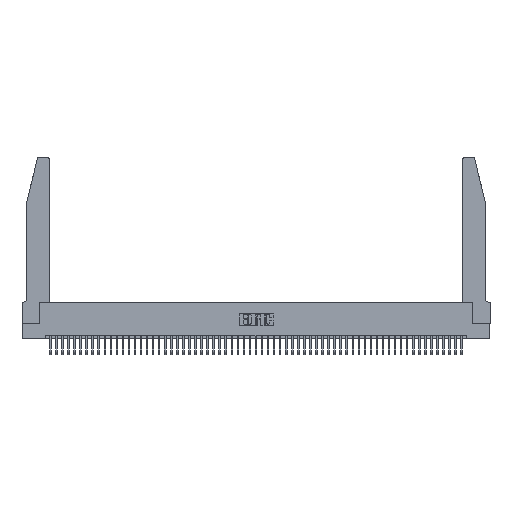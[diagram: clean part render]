
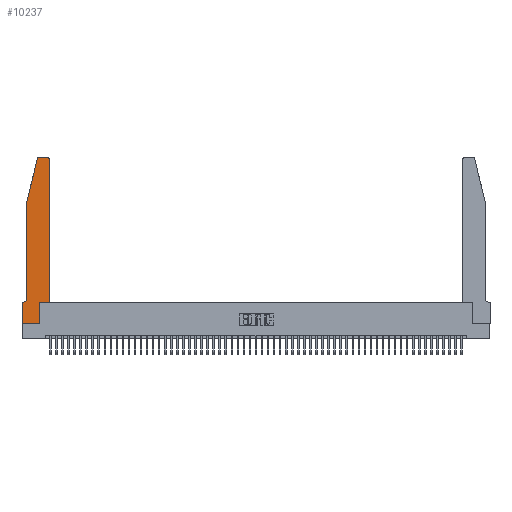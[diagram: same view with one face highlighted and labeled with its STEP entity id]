
A CAD part, top view. The second image highlights one B-rep face of the part: STEP entity #10237.
In plain terms, the highlighted planar face has unit normal (0, 0, 1).
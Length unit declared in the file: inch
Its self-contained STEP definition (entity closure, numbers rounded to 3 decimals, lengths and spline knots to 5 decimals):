
#79 = AXIS2_PLACEMENT_3D ( 'NONE', #24327, #52691, #28423 ) ;
#608 = DIRECTION ( 'NONE',  ( 1., 0., 0. ) ) ;
#946 = DIRECTION ( 'NONE',  ( -1., 0., 0. ) ) ;
#1946 = VERTEX_POINT ( 'NONE', #51150 ) ;
#1989 = EDGE_CURVE ( 'NONE', #50566, #15829, #42300, .T. ) ;
#2062 = VERTEX_POINT ( 'NONE', #47777 ) ;
#3267 = CIRCLE ( 'NONE', #79, 0.03 ) ;
#3657 = VERTEX_POINT ( 'NONE', #42501 ) ;
#4906 = LINE ( 'NONE', #50352, #36424 ) ;
#5288 = VERTEX_POINT ( 'NONE', #52669 ) ;
#5854 = VECTOR ( 'NONE', #33535, 39.37008 ) ;
#5863 = LINE ( 'NONE', #35959, #27805 ) ;
#6526 = VECTOR ( 'NONE', #21671, 39.37008 ) ;
#8458 = ORIENTED_EDGE ( 'NONE', *, *, #50319, .T. ) ;
#8859 = CARTESIAN_POINT ( 'NONE',  ( 0.4205, 2.72, 0.37 ) ) ;
#9174 = CIRCLE ( 'NONE', #15406, 0.07 ) ;
#9323 = EDGE_CURVE ( 'NONE', #41227, #2062, #26548, .T. ) ;
#10237 = ADVANCED_FACE ( 'NONE', ( #10332 ), #19531, .T. ) ;
#10332 = FACE_OUTER_BOUND ( 'NONE', #48337, .T. ) ;
#10875 = VERTEX_POINT ( 'NONE', #20362 ) ;
#11141 = ORIENTED_EDGE ( 'NONE', *, *, #15464, .T. ) ;
#11398 = DIRECTION ( 'NONE',  ( 0., 1., 0. ) ) ;
#11643 = AXIS2_PLACEMENT_3D ( 'NONE', #39808, #47992, #23656 ) ;
#11750 = VECTOR ( 'NONE', #25500, 39.37008 ) ;
#12525 = DIRECTION ( 'NONE',  ( -1., 0., 0. ) ) ;
#13032 = DIRECTION ( 'NONE',  ( 1., 0., 0. ) ) ;
#13220 = CARTESIAN_POINT ( 'NONE',  ( 0., 0., 0.37 ) ) ;
#13730 = ORIENTED_EDGE ( 'NONE', *, *, #23827, .T. ) ;
#13748 = CARTESIAN_POINT ( 'NONE',  ( 0.2865, 0.35, 0.37 ) ) ;
#14004 = VERTEX_POINT ( 'NONE', #48179 ) ;
#15406 = AXIS2_PLACEMENT_3D ( 'NONE', #50113, #25794, #946 ) ;
#15464 = EDGE_CURVE ( 'NONE', #15829, #14004, #43086, .T. ) ;
#15829 = VERTEX_POINT ( 'NONE', #23477 ) ;
#15994 = VECTOR ( 'NONE', #12525, 39.37008 ) ;
#17924 = ORIENTED_EDGE ( 'NONE', *, *, #21934, .T. ) ;
#18050 = ORIENTED_EDGE ( 'NONE', *, *, #23444, .T. ) ;
#18974 = DIRECTION ( 'NONE',  ( -0.239, -0.971, 0. ) ) ;
#19460 = VECTOR ( 'NONE', #608, 39.37008 ) ;
#19531 = PLANE ( 'NONE',  #11643 ) ;
#20362 = CARTESIAN_POINT ( 'NONE',  ( 0.4505, 0.35, 0.37 ) ) ;
#21551 = ORIENTED_EDGE ( 'NONE', *, *, #1989, .T. ) ;
#21671 = DIRECTION ( 'NONE',  ( 1., 0., 0. ) ) ;
#21898 = EDGE_CURVE ( 'NONE', #14004, #5288, #9174, .T. ) ;
#21934 = EDGE_CURVE ( 'NONE', #38759, #10875, #27206, .T. ) ;
#23444 = EDGE_CURVE ( 'NONE', #10875, #1946, #5863, .T. ) ;
#23477 = CARTESIAN_POINT ( 'NONE',  ( 0.0755, 2., 0.37 ) ) ;
#23656 = DIRECTION ( 'NONE',  ( 1., 0., 0. ) ) ;
#23791 = ORIENTED_EDGE ( 'NONE', *, *, #50765, .T. ) ;
#23827 = EDGE_CURVE ( 'NONE', #29746, #38759, #30317, .T. ) ;
#24327 = CARTESIAN_POINT ( 'NONE',  ( 0.284, 2.72, 0.37 ) ) ;
#24473 = VERTEX_POINT ( 'NONE', #26103 ) ;
#25329 = CARTESIAN_POINT ( 'NONE',  ( 0.0755, 2., 0.37 ) ) ;
#25500 = DIRECTION ( 'NONE',  ( 0., -1., 0. ) ) ;
#25794 = DIRECTION ( 'NONE',  ( 0., 0., -1. ) ) ;
#26103 = CARTESIAN_POINT ( 'NONE',  ( 0.284, 2.75, 0.37 ) ) ;
#26548 = LINE ( 'NONE', #49807, #5854 ) ;
#27206 = LINE ( 'NONE', #46211, #6526 ) ;
#27805 = VECTOR ( 'NONE', #11398, 39.37008 ) ;
#28143 = CARTESIAN_POINT ( 'NONE',  ( 0.2865, 0.35, 0.37 ) ) ;
#28184 = LINE ( 'NONE', #45191, #15994 ) ;
#28423 = DIRECTION ( 'NONE',  ( 1., 0., 0. ) ) ;
#28723 = AXIS2_PLACEMENT_3D ( 'NONE', #8859, #37577, #13032 ) ;
#28855 = EDGE_CURVE ( 'NONE', #1946, #3657, #44940, .T. ) ;
#29068 = VECTOR ( 'NONE', #38255, 39.37008 ) ;
#29746 = VERTEX_POINT ( 'NONE', #38702 ) ;
#30317 = LINE ( 'NONE', #13748, #29068 ) ;
#33535 = DIRECTION ( 'NONE',  ( 0., -1., 0. ) ) ;
#34513 = EDGE_CURVE ( 'NONE', #24473, #50566, #3267, .T. ) ;
#34666 = ORIENTED_EDGE ( 'NONE', *, *, #9323, .T. ) ;
#34833 = ORIENTED_EDGE ( 'NONE', *, *, #28855, .T. ) ;
#35959 = CARTESIAN_POINT ( 'NONE',  ( 0.4505, 0.35, 0.37 ) ) ;
#36424 = VECTOR ( 'NONE', #38319, 39.37008 ) ;
#37577 = DIRECTION ( 'NONE',  ( 0., 0., 1. ) ) ;
#38255 = DIRECTION ( 'NONE',  ( 0., 1., 0. ) ) ;
#38319 = DIRECTION ( 'NONE',  ( -1., 0., 0. ) ) ;
#38702 = CARTESIAN_POINT ( 'NONE',  ( 0.2865, 0., 0.37 ) ) ;
#38759 = VERTEX_POINT ( 'NONE', #28143 ) ;
#39274 = CARTESIAN_POINT ( 'NONE',  ( 0.0755, 2., 0.37 ) ) ;
#39808 = CARTESIAN_POINT ( 'NONE',  ( 0., 0.35, 0.37 ) ) ;
#40567 = ORIENTED_EDGE ( 'NONE', *, *, #21898, .T. ) ;
#41132 = LINE ( 'NONE', #13220, #19460 ) ;
#41227 = VERTEX_POINT ( 'NONE', #46007 ) ;
#42300 = LINE ( 'NONE', #39274, #53055 ) ;
#42501 = CARTESIAN_POINT ( 'NONE',  ( 0.4205, 2.75, 0.37 ) ) ;
#42677 = EDGE_CURVE ( 'NONE', #2062, #29746, #41132, .T. ) ;
#43086 = LINE ( 'NONE', #25329, #11750 ) ;
#43131 = ORIENTED_EDGE ( 'NONE', *, *, #34513, .T. ) ;
#44940 = CIRCLE ( 'NONE', #28723, 0.03 ) ;
#45058 = CARTESIAN_POINT ( 'NONE',  ( 0.25487, 2.72718, 0.37 ) ) ;
#45191 = CARTESIAN_POINT ( 'NONE',  ( 0.2605, 2.75, 0.37 ) ) ;
#46007 = CARTESIAN_POINT ( 'NONE',  ( 0., 0.35, 0.37 ) ) ;
#46014 = ORIENTED_EDGE ( 'NONE', *, *, #42677, .T. ) ;
#46211 = CARTESIAN_POINT ( 'NONE',  ( 0.4505, 0.35, 0.37 ) ) ;
#47777 = CARTESIAN_POINT ( 'NONE',  ( 0., 0., 0.37 ) ) ;
#47992 = DIRECTION ( 'NONE',  ( 0., 0., 1. ) ) ;
#48179 = CARTESIAN_POINT ( 'NONE',  ( 0.0755, 0.42, 0.37 ) ) ;
#48337 = EDGE_LOOP ( 'NONE', ( #8458, #43131, #21551, #11141, #40567, #23791, #34666, #46014, #13730, #17924, #18050, #34833 ) ) ;
#49807 = CARTESIAN_POINT ( 'NONE',  ( 0., 0., 0.37 ) ) ;
#50113 = CARTESIAN_POINT ( 'NONE',  ( 0.0055, 0.42, 0.37 ) ) ;
#50319 = EDGE_CURVE ( 'NONE', #3657, #24473, #28184, .T. ) ;
#50352 = CARTESIAN_POINT ( 'NONE',  ( 0.0755, 0.35, 0.37 ) ) ;
#50566 = VERTEX_POINT ( 'NONE', #45058 ) ;
#50765 = EDGE_CURVE ( 'NONE', #5288, #41227, #4906, .T. ) ;
#51150 = CARTESIAN_POINT ( 'NONE',  ( 0.4505, 2.72, 0.37 ) ) ;
#52669 = CARTESIAN_POINT ( 'NONE',  ( 0.0055, 0.35, 0.37 ) ) ;
#52691 = DIRECTION ( 'NONE',  ( 0., 0., 1. ) ) ;
#53055 = VECTOR ( 'NONE', #18974, 39.37008 ) ;
